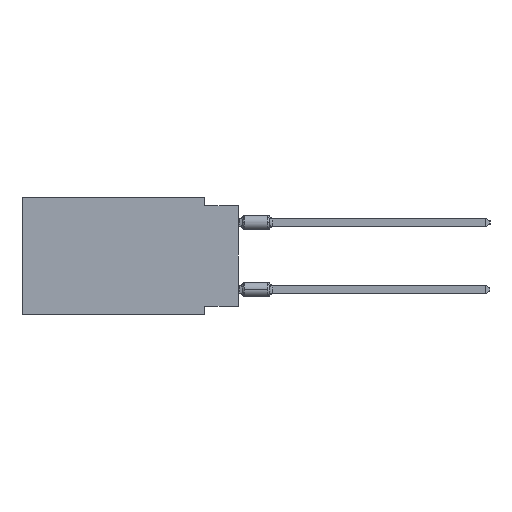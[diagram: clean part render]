
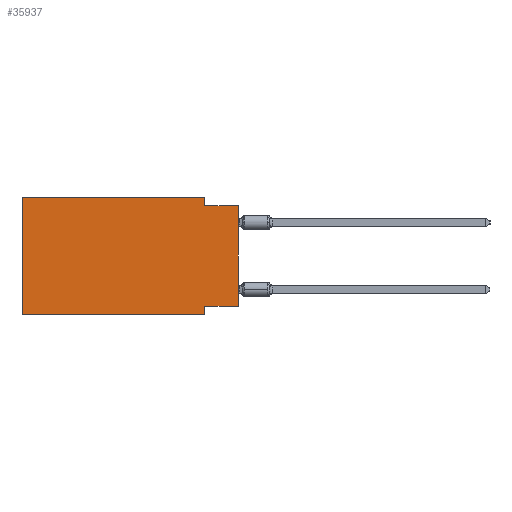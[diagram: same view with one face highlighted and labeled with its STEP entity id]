
A CAD part, left-side view. The second image highlights one B-rep face of the part: STEP entity #35937.
In plain terms, the highlighted planar face has unit normal (-1, 0, 0).
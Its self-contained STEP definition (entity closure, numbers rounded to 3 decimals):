
#166 = EDGE_CURVE ( 'NONE', #2927, #15810, #6150, .T. ) ;
#893 = LINE ( 'NONE', #23556, #16150 ) ;
#1887 = DIRECTION ( 'NONE',  ( 0., 0., 1. ) ) ;
#2375 = CARTESIAN_POINT ( 'NONE',  ( 0., 2.54, 0. ) ) ;
#2743 = CARTESIAN_POINT ( 'NONE',  ( 0., 0., -0.635 ) ) ;
#2809 = LINE ( 'NONE', #14505, #4012 ) ;
#2927 = VERTEX_POINT ( 'NONE', #29457 ) ;
#2939 = DIRECTION ( 'NONE',  ( 0., 0., -1. ) ) ;
#3270 = EDGE_CURVE ( 'NONE', #15077, #15810, #893, .T. ) ;
#3273 = CARTESIAN_POINT ( 'NONE',  ( 0., 2.54, -0.635 ) ) ;
#3554 = EDGE_CURVE ( 'NONE', #21097, #26267, #19747, .T. ) ;
#4012 = VECTOR ( 'NONE', #23188, 1000. ) ;
#4151 = VERTEX_POINT ( 'NONE', #2743 ) ;
#4823 = CARTESIAN_POINT ( 'NONE',  ( 0., 2.54, -8.255 ) ) ;
#4944 = EDGE_CURVE ( 'NONE', #29007, #15077, #25097, .T. ) ;
#5625 = LINE ( 'NONE', #34147, #23302 ) ;
#6150 = LINE ( 'NONE', #19956, #28768 ) ;
#7629 = PLANE ( 'NONE',  #36385 ) ;
#8067 = DIRECTION ( 'NONE',  ( 0., 1., 0. ) ) ;
#11123 = VECTOR ( 'NONE', #29194, 1000. ) ;
#11822 = VECTOR ( 'NONE', #1887, 1000. ) ;
#13567 = EDGE_CURVE ( 'NONE', #29007, #4151, #33793, .T. ) ;
#14505 = CARTESIAN_POINT ( 'NONE',  ( 0., 16.383, 0. ) ) ;
#14932 = ORIENTED_EDGE ( 'NONE', *, *, #13567, .T. ) ;
#15077 = VERTEX_POINT ( 'NONE', #4823 ) ;
#15810 = VERTEX_POINT ( 'NONE', #28930 ) ;
#16150 = VECTOR ( 'NONE', #18248, 1000. ) ;
#16405 = ORIENTED_EDGE ( 'NONE', *, *, #3554, .F. ) ;
#16684 = FACE_OUTER_BOUND ( 'NONE', #25813, .T. ) ;
#16993 = ORIENTED_EDGE ( 'NONE', *, *, #166, .T. ) ;
#17496 = DIRECTION ( 'NONE',  ( 0., -1., 0. ) ) ;
#18060 = EDGE_CURVE ( 'NONE', #33347, #21097, #37310, .T. ) ;
#18248 = DIRECTION ( 'NONE',  ( 0., 0., -1. ) ) ;
#19747 = LINE ( 'NONE', #2375, #36673 ) ;
#19956 = CARTESIAN_POINT ( 'NONE',  ( 0., 16.383, -8.89 ) ) ;
#21097 = VERTEX_POINT ( 'NONE', #29505 ) ;
#21842 = ORIENTED_EDGE ( 'NONE', *, *, #24251, .F. ) ;
#22351 = CARTESIAN_POINT ( 'NONE',  ( 0., 16.383, 0. ) ) ;
#22431 = DIRECTION ( 'NONE',  ( 0., -1., 0. ) ) ;
#23188 = DIRECTION ( 'NONE',  ( 0., 0., 1. ) ) ;
#23302 = VECTOR ( 'NONE', #22431, 1000. ) ;
#23556 = CARTESIAN_POINT ( 'NONE',  ( 0., 2.54, -8.89 ) ) ;
#24251 = EDGE_CURVE ( 'NONE', #26267, #4151, #5625, .T. ) ;
#24302 = EDGE_CURVE ( 'NONE', #2927, #33347, #2809, .T. ) ;
#25097 = LINE ( 'NONE', #36604, #30108 ) ;
#25813 = EDGE_LOOP ( 'NONE', ( #14932, #21842, #16405, #35873, #32848, #16993, #35967, #34457 ) ) ;
#26267 = VERTEX_POINT ( 'NONE', #3273 ) ;
#26678 = CARTESIAN_POINT ( 'NONE',  ( 0., 16.383, 0. ) ) ;
#27296 = CARTESIAN_POINT ( 'NONE',  ( 0., 0., -8.255 ) ) ;
#27764 = CARTESIAN_POINT ( 'NONE',  ( 0., 0., 0. ) ) ;
#28768 = VECTOR ( 'NONE', #17496, 1000. ) ;
#28930 = CARTESIAN_POINT ( 'NONE',  ( 0., 2.54, -8.89 ) ) ;
#29007 = VERTEX_POINT ( 'NONE', #27296 ) ;
#29194 = DIRECTION ( 'NONE',  ( 0., -1., 0. ) ) ;
#29457 = CARTESIAN_POINT ( 'NONE',  ( 0., 16.383, -8.89 ) ) ;
#29505 = CARTESIAN_POINT ( 'NONE',  ( 0., 2.54, 0. ) ) ;
#30108 = VECTOR ( 'NONE', #8067, 1000. ) ;
#32848 = ORIENTED_EDGE ( 'NONE', *, *, #24302, .F. ) ;
#33347 = VERTEX_POINT ( 'NONE', #26678 ) ;
#33690 = DIRECTION ( 'NONE',  ( 1., 0., 0. ) ) ;
#33793 = LINE ( 'NONE', #27764, #11822 ) ;
#34147 = CARTESIAN_POINT ( 'NONE',  ( 0., 0., -0.635 ) ) ;
#34457 = ORIENTED_EDGE ( 'NONE', *, *, #4944, .F. ) ;
#35042 = CARTESIAN_POINT ( 'NONE',  ( 0., 16.383, 0. ) ) ;
#35873 = ORIENTED_EDGE ( 'NONE', *, *, #18060, .F. ) ;
#35937 = ADVANCED_FACE ( 'NONE', ( #16684 ), #7629, .F. ) ;
#35967 = ORIENTED_EDGE ( 'NONE', *, *, #3270, .F. ) ;
#36385 = AXIS2_PLACEMENT_3D ( 'NONE', #22351, #33690, #36518 ) ;
#36518 = DIRECTION ( 'NONE',  ( 0., 0., -1. ) ) ;
#36604 = CARTESIAN_POINT ( 'NONE',  ( 0., 0., -8.255 ) ) ;
#36673 = VECTOR ( 'NONE', #2939, 1000. ) ;
#37310 = LINE ( 'NONE', #35042, #11123 ) ;
